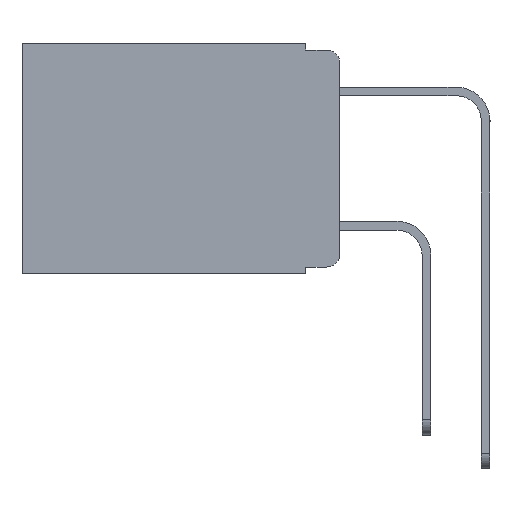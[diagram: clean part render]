
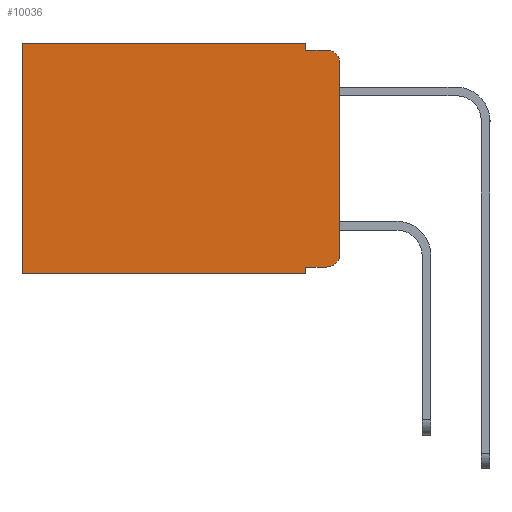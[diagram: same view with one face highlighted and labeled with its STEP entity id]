
A CAD part, left-side view. The second image highlights one B-rep face of the part: STEP entity #10036.
In plain terms, the highlighted planar face has unit normal (-1, 0, 0).
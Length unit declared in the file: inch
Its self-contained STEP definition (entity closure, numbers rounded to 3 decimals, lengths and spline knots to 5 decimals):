
#226 = VECTOR ( 'NONE', #23868, 39.37008 ) ;
#299 = CIRCLE ( 'NONE', #23430, 0.02 ) ;
#332 = ORIENTED_EDGE ( 'NONE', *, *, #22589, .T. ) ;
#1167 = EDGE_CURVE ( 'NONE', #14292, #11131, #18065, .T. ) ;
#1787 = EDGE_CURVE ( 'NONE', #23855, #18083, #26631, .T. ) ;
#2138 = CARTESIAN_POINT ( 'NONE',  ( 0.298, 0., 0. ) ) ;
#2695 = ORIENTED_EDGE ( 'NONE', *, *, #9075, .F. ) ;
#3824 = CARTESIAN_POINT ( 'NONE',  ( 0.298, 0.02, -0.01 ) ) ;
#4006 = CARTESIAN_POINT ( 'NONE',  ( 0.298, 0.051, 0. ) ) ;
#4282 = DIRECTION ( 'NONE',  ( 1., 0., 0. ) ) ;
#4370 = CARTESIAN_POINT ( 'NONE',  ( 0.298, 0., 0. ) ) ;
#4631 = EDGE_CURVE ( 'NONE', #4843, #12731, #8123, .T. ) ;
#4843 = VERTEX_POINT ( 'NONE', #11516 ) ;
#5600 = AXIS2_PLACEMENT_3D ( 'NONE', #2138, #4282, #18846 ) ;
#5925 = LINE ( 'NONE', #7578, #226 ) ;
#6038 = ORIENTED_EDGE ( 'NONE', *, *, #12820, .F. ) ;
#6697 = ORIENTED_EDGE ( 'NONE', *, *, #10950, .T. ) ;
#7031 = ORIENTED_EDGE ( 'NONE', *, *, #4631, .T. ) ;
#7361 = CARTESIAN_POINT ( 'NONE',  ( 0.298, 0.02, -0.313 ) ) ;
#7524 = DIRECTION ( 'NONE',  ( 0., 0., -1. ) ) ;
#7578 = CARTESIAN_POINT ( 'NONE',  ( 0.298, 0.051, -0.01 ) ) ;
#7594 = EDGE_LOOP ( 'NONE', ( #12627, #7031, #2695, #12308, #6697, #332, #21208, #6038, #17763, #8031 ) ) ;
#7644 = VECTOR ( 'NONE', #7524, 39.37008 ) ;
#7664 = EDGE_CURVE ( 'NONE', #11131, #11606, #299, .T. ) ;
#7751 = VECTOR ( 'NONE', #24095, 39.37008 ) ;
#8031 = ORIENTED_EDGE ( 'NONE', *, *, #7664, .T. ) ;
#8123 = CIRCLE ( 'NONE', #12238, 0.02 ) ;
#8590 = LINE ( 'NONE', #19397, #12860 ) ;
#8761 = CARTESIAN_POINT ( 'NONE',  ( 0.298, 0.02, -0.03 ) ) ;
#8917 = EDGE_CURVE ( 'NONE', #4843, #11606, #9932, .T. ) ;
#9075 = EDGE_CURVE ( 'NONE', #18083, #12731, #5925, .T. ) ;
#9136 = DIRECTION ( 'NONE',  ( 0., 1., 0. ) ) ;
#9289 = CARTESIAN_POINT ( 'NONE',  ( 0.298, 0.02, -0.333 ) ) ;
#9512 = DIRECTION ( 'NONE',  ( 0., 0., -1. ) ) ;
#9588 = VECTOR ( 'NONE', #16504, 39.37008 ) ;
#9794 = CARTESIAN_POINT ( 'NONE',  ( 0.298, 0.051, -0.333 ) ) ;
#9932 = LINE ( 'NONE', #17403, #14782 ) ;
#10036 = ADVANCED_FACE ( 'NONE', ( #10849 ), #14753, .F. ) ;
#10543 = VERTEX_POINT ( 'NONE', #23594 ) ;
#10849 = FACE_OUTER_BOUND ( 'NONE', #7594, .T. ) ;
#10950 = EDGE_CURVE ( 'NONE', #23855, #17671, #17764, .T. ) ;
#11131 = VERTEX_POINT ( 'NONE', #9289 ) ;
#11516 = CARTESIAN_POINT ( 'NONE',  ( 0.298, 0., -0.03 ) ) ;
#11606 = VERTEX_POINT ( 'NONE', #24844 ) ;
#12238 = AXIS2_PLACEMENT_3D ( 'NONE', #8761, #25257, #13271 ) ;
#12308 = ORIENTED_EDGE ( 'NONE', *, *, #1787, .F. ) ;
#12612 = VECTOR ( 'NONE', #19344, 39.37008 ) ;
#12627 = ORIENTED_EDGE ( 'NONE', *, *, #8917, .F. ) ;
#12709 = VERTEX_POINT ( 'NONE', #26217 ) ;
#12731 = VERTEX_POINT ( 'NONE', #3824 ) ;
#12820 = EDGE_CURVE ( 'NONE', #14292, #12709, #26285, .T. ) ;
#12860 = VECTOR ( 'NONE', #9136, 39.37008 ) ;
#13271 = DIRECTION ( 'NONE',  ( 0., 0., -1. ) ) ;
#14292 = VERTEX_POINT ( 'NONE', #17306 ) ;
#14753 = PLANE ( 'NONE',  #5600 ) ;
#14782 = VECTOR ( 'NONE', #21429, 39.37008 ) ;
#16441 = CARTESIAN_POINT ( 'NONE',  ( 0.298, 0.051, -0.01 ) ) ;
#16504 = DIRECTION ( 'NONE',  ( 0., 0., -1. ) ) ;
#16876 = DIRECTION ( 'NONE',  ( 0., 1., 0. ) ) ;
#17300 = CARTESIAN_POINT ( 'NONE',  ( 0.298, 0.473, 0. ) ) ;
#17306 = CARTESIAN_POINT ( 'NONE',  ( 0.298, 0.051, -0.333 ) ) ;
#17403 = CARTESIAN_POINT ( 'NONE',  ( 0.298, 0., 0. ) ) ;
#17671 = VERTEX_POINT ( 'NONE', #17300 ) ;
#17763 = ORIENTED_EDGE ( 'NONE', *, *, #1167, .T. ) ;
#17764 = LINE ( 'NONE', #4370, #24878 ) ;
#18065 = LINE ( 'NONE', #9794, #12612 ) ;
#18083 = VERTEX_POINT ( 'NONE', #16441 ) ;
#18160 = CARTESIAN_POINT ( 'NONE',  ( 0.298, 0.473, 0. ) ) ;
#18712 = CARTESIAN_POINT ( 'NONE',  ( 0.298, 0.051, 0. ) ) ;
#18846 = DIRECTION ( 'NONE',  ( 0., 0., -1. ) ) ;
#19344 = DIRECTION ( 'NONE',  ( 0., -1., 0. ) ) ;
#19397 = CARTESIAN_POINT ( 'NONE',  ( 0.298, 0., -0.343 ) ) ;
#20662 = LINE ( 'NONE', #18160, #7751 ) ;
#20734 = CARTESIAN_POINT ( 'NONE',  ( 0.298, 0.051, 0. ) ) ;
#21208 = ORIENTED_EDGE ( 'NONE', *, *, #25614, .F. ) ;
#21429 = DIRECTION ( 'NONE',  ( 0., 0., -1. ) ) ;
#21726 = DIRECTION ( 'NONE',  ( -1., 0., 0. ) ) ;
#22589 = EDGE_CURVE ( 'NONE', #17671, #10543, #20662, .T. ) ;
#23430 = AXIS2_PLACEMENT_3D ( 'NONE', #7361, #21726, #9512 ) ;
#23594 = CARTESIAN_POINT ( 'NONE',  ( 0.298, 0.473, -0.343 ) ) ;
#23855 = VERTEX_POINT ( 'NONE', #20734 ) ;
#23868 = DIRECTION ( 'NONE',  ( 0., -1., 0. ) ) ;
#24095 = DIRECTION ( 'NONE',  ( 0., 0., -1. ) ) ;
#24844 = CARTESIAN_POINT ( 'NONE',  ( 0.298, 0., -0.313 ) ) ;
#24878 = VECTOR ( 'NONE', #16876, 39.37008 ) ;
#25257 = DIRECTION ( 'NONE',  ( -1., 0., 0. ) ) ;
#25614 = EDGE_CURVE ( 'NONE', #12709, #10543, #8590, .T. ) ;
#26217 = CARTESIAN_POINT ( 'NONE',  ( 0.298, 0.051, -0.343 ) ) ;
#26285 = LINE ( 'NONE', #4006, #9588 ) ;
#26631 = LINE ( 'NONE', #18712, #7644 ) ;
